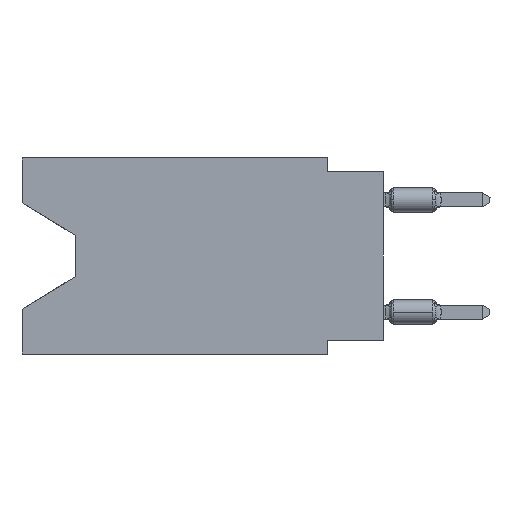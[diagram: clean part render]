
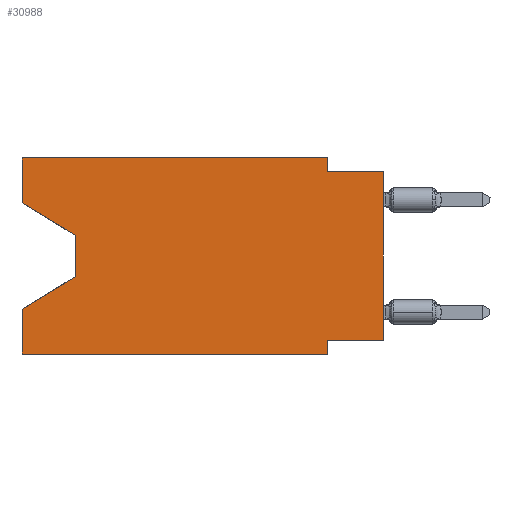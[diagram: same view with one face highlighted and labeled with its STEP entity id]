
A CAD part, left-side view. The second image highlights one B-rep face of the part: STEP entity #30988.
In plain terms, the highlighted planar face has unit normal (-1, 0, 0).
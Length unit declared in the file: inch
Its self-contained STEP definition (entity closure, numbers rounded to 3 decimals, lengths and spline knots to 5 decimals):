
#39 = LINE ( 'NONE', #22281, #71291 ) ;
#2770 = EDGE_CURVE ( 'NONE', #11693, #18123, #39, .T. ) ;
#5100 = LINE ( 'NONE', #21898, #47283 ) ;
#5878 = EDGE_CURVE ( 'NONE', #43080, #26609, #55277, .T. ) ;
#6225 = VECTOR ( 'NONE', #30171, 39.37008 ) ;
#7438 = CARTESIAN_POINT ( 'NONE',  ( 0., 0.1, -0.025 ) ) ;
#9652 = ORIENTED_EDGE ( 'NONE', *, *, #32175, .F. ) ;
#9766 = EDGE_CURVE ( 'NONE', #22628, #46086, #52746, .T. ) ;
#11133 = CARTESIAN_POINT ( 'NONE',  ( 0., 0.55, -0.138 ) ) ;
#11693 = VERTEX_POINT ( 'NONE', #7438 ) ;
#12373 = VECTOR ( 'NONE', #64173, 39.37008 ) ;
#13009 = CARTESIAN_POINT ( 'NONE',  ( 0., 0.645, 0. ) ) ;
#13789 = FACE_OUTER_BOUND ( 'NONE', #62586, .T. ) ;
#14469 = EDGE_CURVE ( 'NONE', #35191, #58070, #47648, .T. ) ;
#15128 = CARTESIAN_POINT ( 'NONE',  ( 0., 0.645, 0. ) ) ;
#16646 = CARTESIAN_POINT ( 'NONE',  ( 0., 0.1, -0.35 ) ) ;
#17291 = ORIENTED_EDGE ( 'NONE', *, *, #24359, .F. ) ;
#17412 = ORIENTED_EDGE ( 'NONE', *, *, #5878, .F. ) ;
#17739 = VERTEX_POINT ( 'NONE', #64390 ) ;
#18123 = VERTEX_POINT ( 'NONE', #53973 ) ;
#18716 = LINE ( 'NONE', #40921, #51288 ) ;
#21898 = CARTESIAN_POINT ( 'NONE',  ( 0., 0.645, -0.35 ) ) ;
#22281 = CARTESIAN_POINT ( 'NONE',  ( 0., 0., -0.025 ) ) ;
#22628 = VERTEX_POINT ( 'NONE', #36944 ) ;
#23458 = CARTESIAN_POINT ( 'NONE',  ( 0., 0.645, -0.26975 ) ) ;
#24359 = EDGE_CURVE ( 'NONE', #68957, #17739, #65072, .T. ) ;
#24417 = ORIENTED_EDGE ( 'NONE', *, *, #38980, .F. ) ;
#24706 = DIRECTION ( 'NONE',  ( 0., 0., -1. ) ) ;
#25036 = DIRECTION ( 'NONE',  ( 0., 0., 1. ) ) ;
#26609 = VERTEX_POINT ( 'NONE', #54491 ) ;
#27142 = CARTESIAN_POINT ( 'NONE',  ( 0., 0., -0.325 ) ) ;
#28321 = EDGE_CURVE ( 'NONE', #62862, #43080, #39446, .T. ) ;
#30171 = DIRECTION ( 'NONE',  ( 0., -0.855, -0.519 ) ) ;
#30771 = EDGE_CURVE ( 'NONE', #46086, #63730, #34933, .T. ) ;
#30988 = ADVANCED_FACE ( 'NONE', ( #13789 ), #64096, .F. ) ;
#32110 = VECTOR ( 'NONE', #50590, 39.37008 ) ;
#32130 = DIRECTION ( 'NONE',  ( 0., -1., 0. ) ) ;
#32175 = EDGE_CURVE ( 'NONE', #17739, #11693, #18716, .T. ) ;
#32306 = VECTOR ( 'NONE', #56749, 39.37008 ) ;
#34848 = VECTOR ( 'NONE', #56075, 39.37008 ) ;
#34933 = LINE ( 'NONE', #68475, #34848 ) ;
#35191 = VERTEX_POINT ( 'NONE', #41098 ) ;
#35590 = DIRECTION ( 'NONE',  ( 0., 0., 1. ) ) ;
#36035 = CARTESIAN_POINT ( 'NONE',  ( 0., 0.645, 0. ) ) ;
#36117 = CARTESIAN_POINT ( 'NONE',  ( 0., 0.645, 0. ) ) ;
#36467 = ORIENTED_EDGE ( 'NONE', *, *, #37063, .T. ) ;
#36944 = CARTESIAN_POINT ( 'NONE',  ( 0., 0.645, -0.08025 ) ) ;
#37049 = ORIENTED_EDGE ( 'NONE', *, *, #9766, .T. ) ;
#37063 = EDGE_CURVE ( 'NONE', #63730, #58070, #57145, .T. ) ;
#37844 = CARTESIAN_POINT ( 'NONE',  ( 0., 0.645, 0. ) ) ;
#38980 = EDGE_CURVE ( 'NONE', #22628, #68957, #69661, .T. ) ;
#39446 = LINE ( 'NONE', #50337, #51680 ) ;
#39579 = ORIENTED_EDGE ( 'NONE', *, *, #14469, .F. ) ;
#40683 = AXIS2_PLACEMENT_3D ( 'NONE', #36035, #58263, #24706 ) ;
#40921 = CARTESIAN_POINT ( 'NONE',  ( 0., 0.1, 0. ) ) ;
#41076 = CARTESIAN_POINT ( 'NONE',  ( 0., 0.645, -0.08025 ) ) ;
#41098 = CARTESIAN_POINT ( 'NONE',  ( 0., 0.645, -0.35 ) ) ;
#41215 = ORIENTED_EDGE ( 'NONE', *, *, #2770, .F. ) ;
#43080 = VERTEX_POINT ( 'NONE', #71204 ) ;
#44529 = DIRECTION ( 'NONE',  ( 0., -1., 0. ) ) ;
#44940 = EDGE_CURVE ( 'NONE', #35191, #26609, #5100, .T. ) ;
#45064 = ORIENTED_EDGE ( 'NONE', *, *, #61719, .T. ) ;
#46086 = VERTEX_POINT ( 'NONE', #11133 ) ;
#46878 = CARTESIAN_POINT ( 'NONE',  ( 0., 0., 0. ) ) ;
#47283 = VECTOR ( 'NONE', #32130, 39.37008 ) ;
#47648 = LINE ( 'NONE', #13009, #55471 ) ;
#50337 = CARTESIAN_POINT ( 'NONE',  ( 0., 0., -0.325 ) ) ;
#50590 = DIRECTION ( 'NONE',  ( 0., 0.855, -0.519 ) ) ;
#51288 = VECTOR ( 'NONE', #63161, 39.37008 ) ;
#51429 = DIRECTION ( 'NONE',  ( 0., 1., 0. ) ) ;
#51680 = VECTOR ( 'NONE', #51429, 39.37008 ) ;
#52746 = LINE ( 'NONE', #41076, #6225 ) ;
#53785 = VECTOR ( 'NONE', #65664, 39.37008 ) ;
#53973 = CARTESIAN_POINT ( 'NONE',  ( 0., 0., -0.025 ) ) ;
#54491 = CARTESIAN_POINT ( 'NONE',  ( 0., 0.1, -0.35 ) ) ;
#55277 = LINE ( 'NONE', #16646, #32306 ) ;
#55412 = CARTESIAN_POINT ( 'NONE',  ( 0., 0.55, -0.212 ) ) ;
#55471 = VECTOR ( 'NONE', #25036, 39.37008 ) ;
#56075 = DIRECTION ( 'NONE',  ( 0., 0., -1. ) ) ;
#56626 = ORIENTED_EDGE ( 'NONE', *, *, #30771, .T. ) ;
#56749 = DIRECTION ( 'NONE',  ( 0., 0., -1. ) ) ;
#57100 = LINE ( 'NONE', #46878, #63516 ) ;
#57145 = LINE ( 'NONE', #62983, #32110 ) ;
#58070 = VERTEX_POINT ( 'NONE', #23458 ) ;
#58263 = DIRECTION ( 'NONE',  ( 1., 0., 0. ) ) ;
#61719 = EDGE_CURVE ( 'NONE', #62862, #18123, #57100, .T. ) ;
#62586 = EDGE_LOOP ( 'NONE', ( #37049, #56626, #36467, #39579, #63118, #17412, #69925, #45064, #41215, #9652, #17291, #24417 ) ) ;
#62862 = VERTEX_POINT ( 'NONE', #27142 ) ;
#62983 = CARTESIAN_POINT ( 'NONE',  ( 0., 0.55, -0.212 ) ) ;
#63118 = ORIENTED_EDGE ( 'NONE', *, *, #44940, .T. ) ;
#63161 = DIRECTION ( 'NONE',  ( 0., 0., -1. ) ) ;
#63516 = VECTOR ( 'NONE', #35590, 39.37008 ) ;
#63730 = VERTEX_POINT ( 'NONE', #55412 ) ;
#64096 = PLANE ( 'NONE',  #40683 ) ;
#64173 = DIRECTION ( 'NONE',  ( 0., 0., 1. ) ) ;
#64390 = CARTESIAN_POINT ( 'NONE',  ( 0., 0.1, 0. ) ) ;
#65072 = LINE ( 'NONE', #15128, #53785 ) ;
#65664 = DIRECTION ( 'NONE',  ( 0., -1., 0. ) ) ;
#68475 = CARTESIAN_POINT ( 'NONE',  ( 0., 0.55, -0.138 ) ) ;
#68957 = VERTEX_POINT ( 'NONE', #37844 ) ;
#69661 = LINE ( 'NONE', #36117, #12373 ) ;
#69925 = ORIENTED_EDGE ( 'NONE', *, *, #28321, .F. ) ;
#71204 = CARTESIAN_POINT ( 'NONE',  ( 0., 0.1, -0.325 ) ) ;
#71291 = VECTOR ( 'NONE', #44529, 39.37008 ) ;
